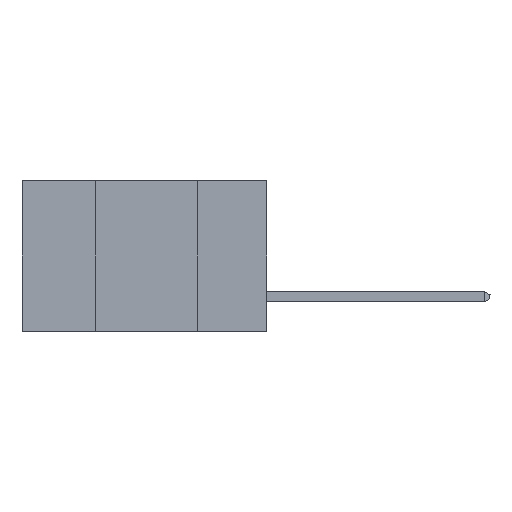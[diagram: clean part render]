
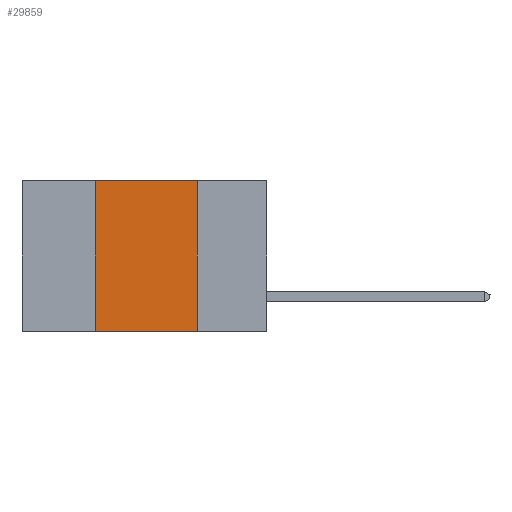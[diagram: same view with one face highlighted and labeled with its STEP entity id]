
A CAD part, left-side view. The second image highlights one B-rep face of the part: STEP entity #29859.
In plain terms, the highlighted planar face has unit normal (-1, 0, 0).
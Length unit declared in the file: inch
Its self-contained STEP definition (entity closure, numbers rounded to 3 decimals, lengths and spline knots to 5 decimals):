
#2194 = ORIENTED_EDGE ( 'NONE', *, *, #26446, .F. ) ;
#5475 = FACE_OUTER_BOUND ( 'NONE', #21645, .T. ) ;
#6012 = ORIENTED_EDGE ( 'NONE', *, *, #45113, .F. ) ;
#7575 = CARTESIAN_POINT ( 'NONE',  ( 0., 0.6, 0. ) ) ;
#7610 = LINE ( 'NONE', #43817, #25903 ) ;
#9332 = EDGE_CURVE ( 'NONE', #14553, #34706, #12021, .T. ) ;
#9541 = EDGE_CURVE ( 'NONE', #25019, #34706, #11571, .T. ) ;
#11571 = LINE ( 'NONE', #14374, #41527 ) ;
#12021 = LINE ( 'NONE', #12713, #42414 ) ;
#12713 = CARTESIAN_POINT ( 'NONE',  ( 0., 0.6, -0.37 ) ) ;
#12722 = ORIENTED_EDGE ( 'NONE', *, *, #9332, .T. ) ;
#12803 = CARTESIAN_POINT ( 'NONE',  ( 0., 0.42, 0. ) ) ;
#14106 = CARTESIAN_POINT ( 'NONE',  ( 0., 0.42, -0.37 ) ) ;
#14374 = CARTESIAN_POINT ( 'NONE',  ( 0., 0.17, 0. ) ) ;
#14553 = VERTEX_POINT ( 'NONE', #14106 ) ;
#16000 = PLANE ( 'NONE',  #44109 ) ;
#20288 = DIRECTION ( 'NONE',  ( 0., -1., 0. ) ) ;
#21340 = LINE ( 'NONE', #7575, #44035 ) ;
#21645 = EDGE_LOOP ( 'NONE', ( #40574, #6012, #2194, #12722 ) ) ;
#22033 = CARTESIAN_POINT ( 'NONE',  ( 0., 0.17, -0.37 ) ) ;
#23223 = CARTESIAN_POINT ( 'NONE',  ( 0., 0.17, 0. ) ) ;
#25019 = VERTEX_POINT ( 'NONE', #23223 ) ;
#25903 = VECTOR ( 'NONE', #36261, 39.37008 ) ;
#26103 = DIRECTION ( 'NONE',  ( 1., 0., 0. ) ) ;
#26446 = EDGE_CURVE ( 'NONE', #14553, #28264, #7610, .T. ) ;
#28264 = VERTEX_POINT ( 'NONE', #12803 ) ;
#29859 = ADVANCED_FACE ( 'NONE', ( #5475 ), #16000, .F. ) ;
#32349 = DIRECTION ( 'NONE',  ( 0., -1., 0. ) ) ;
#34706 = VERTEX_POINT ( 'NONE', #22033 ) ;
#36261 = DIRECTION ( 'NONE',  ( 0., 0., 1. ) ) ;
#39181 = DIRECTION ( 'NONE',  ( 0., 0., -1. ) ) ;
#40574 = ORIENTED_EDGE ( 'NONE', *, *, #9541, .F. ) ;
#41527 = VECTOR ( 'NONE', #39181, 39.37008 ) ;
#42414 = VECTOR ( 'NONE', #20288, 39.37008 ) ;
#43817 = CARTESIAN_POINT ( 'NONE',  ( 0., 0.42, 0. ) ) ;
#43899 = CARTESIAN_POINT ( 'NONE',  ( 0., 0.6, 0. ) ) ;
#44035 = VECTOR ( 'NONE', #32349, 39.37008 ) ;
#44039 = DIRECTION ( 'NONE',  ( 0., 0., -1. ) ) ;
#44109 = AXIS2_PLACEMENT_3D ( 'NONE', #43899, #26103, #44039 ) ;
#45113 = EDGE_CURVE ( 'NONE', #28264, #25019, #21340, .T. ) ;
